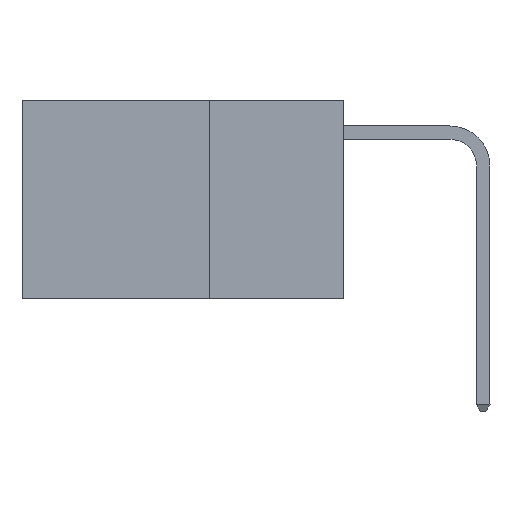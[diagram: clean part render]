
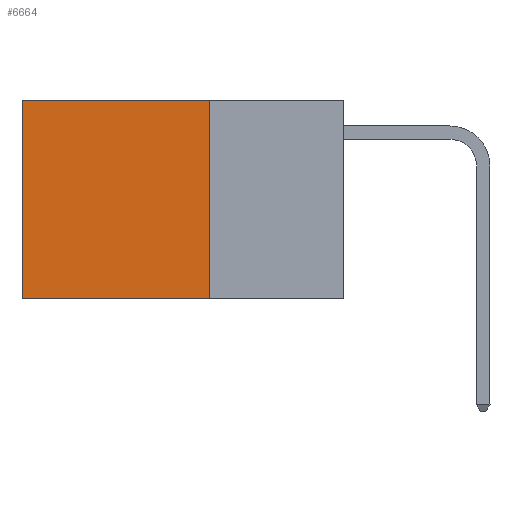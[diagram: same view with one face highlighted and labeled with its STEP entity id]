
A CAD part, left-side view. The second image highlights one B-rep face of the part: STEP entity #6664.
In plain terms, the highlighted planar face has unit normal (-1, 0, 0).
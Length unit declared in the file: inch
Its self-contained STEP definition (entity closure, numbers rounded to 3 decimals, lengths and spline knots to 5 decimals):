
#34 = VERTEX_POINT ( 'NONE', #4391 ) ;
#128 = LINE ( 'NONE', #9261, #8202 ) ;
#202 = PLANE ( 'NONE',  #2425 ) ;
#256 = EDGE_CURVE ( 'NONE', #34, #8808, #128, .T. ) ;
#1295 = ORIENTED_EDGE ( 'NONE', *, *, #2367, .F. ) ;
#1340 = VECTOR ( 'NONE', #3938, 39.37008 ) ;
#1342 = EDGE_CURVE ( 'NONE', #8808, #7146, #3381, .T. ) ;
#1709 = DIRECTION ( 'NONE',  ( 0., 1., 0. ) ) ;
#1741 = DIRECTION ( 'NONE',  ( 0., 0., -1. ) ) ;
#2042 = ORIENTED_EDGE ( 'NONE', *, *, #256, .T. ) ;
#2086 = CARTESIAN_POINT ( 'NONE',  ( 0.2625, 0.6, 0. ) ) ;
#2367 = EDGE_CURVE ( 'NONE', #34, #3842, #6858, .T. ) ;
#2419 = LINE ( 'NONE', #5389, #2546 ) ;
#2425 = AXIS2_PLACEMENT_3D ( 'NONE', #7885, #3223, #1741 ) ;
#2546 = VECTOR ( 'NONE', #8397, 39.37008 ) ;
#3223 = DIRECTION ( 'NONE',  ( 1., 0., 0. ) ) ;
#3298 = CARTESIAN_POINT ( 'NONE',  ( 0.2625, 0.25, -0.37 ) ) ;
#3381 = LINE ( 'NONE', #2086, #5536 ) ;
#3842 = VERTEX_POINT ( 'NONE', #3298 ) ;
#3938 = DIRECTION ( 'NONE',  ( 0., 0., -1. ) ) ;
#4391 = CARTESIAN_POINT ( 'NONE',  ( 0.2625, 0.25, 0. ) ) ;
#5389 = CARTESIAN_POINT ( 'NONE',  ( 0.2625, 0.25, -0.37 ) ) ;
#5536 = VECTOR ( 'NONE', #8801, 39.37008 ) ;
#6664 = ADVANCED_FACE ( 'NONE', ( #7662 ), #202, .F. ) ;
#6724 = EDGE_LOOP ( 'NONE', ( #7818, #9516, #1295, #2042 ) ) ;
#6858 = LINE ( 'NONE', #6908, #1340 ) ;
#6908 = CARTESIAN_POINT ( 'NONE',  ( 0.2625, 0.25, 0. ) ) ;
#7146 = VERTEX_POINT ( 'NONE', #8454 ) ;
#7662 = FACE_OUTER_BOUND ( 'NONE', #6724, .T. ) ;
#7818 = ORIENTED_EDGE ( 'NONE', *, *, #1342, .T. ) ;
#7885 = CARTESIAN_POINT ( 'NONE',  ( 0.2625, 0.25, 0. ) ) ;
#8202 = VECTOR ( 'NONE', #1709, 39.37008 ) ;
#8397 = DIRECTION ( 'NONE',  ( 0., 1., 0. ) ) ;
#8454 = CARTESIAN_POINT ( 'NONE',  ( 0.2625, 0.6, -0.37 ) ) ;
#8557 = EDGE_CURVE ( 'NONE', #3842, #7146, #2419, .T. ) ;
#8801 = DIRECTION ( 'NONE',  ( 0., 0., -1. ) ) ;
#8808 = VERTEX_POINT ( 'NONE', #9190 ) ;
#9190 = CARTESIAN_POINT ( 'NONE',  ( 0.2625, 0.6, 0. ) ) ;
#9261 = CARTESIAN_POINT ( 'NONE',  ( 0.2625, 0.25, 0. ) ) ;
#9516 = ORIENTED_EDGE ( 'NONE', *, *, #8557, .F. ) ;
